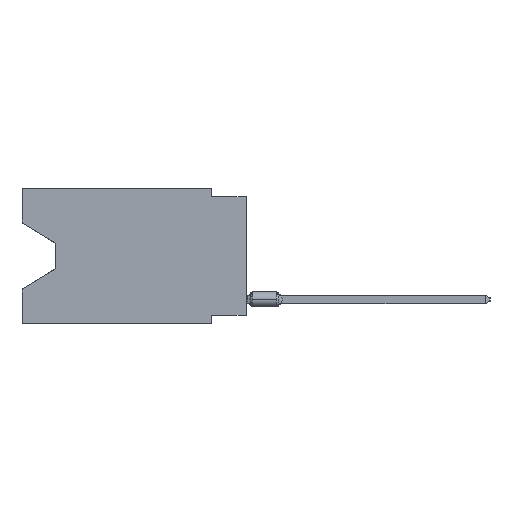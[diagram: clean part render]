
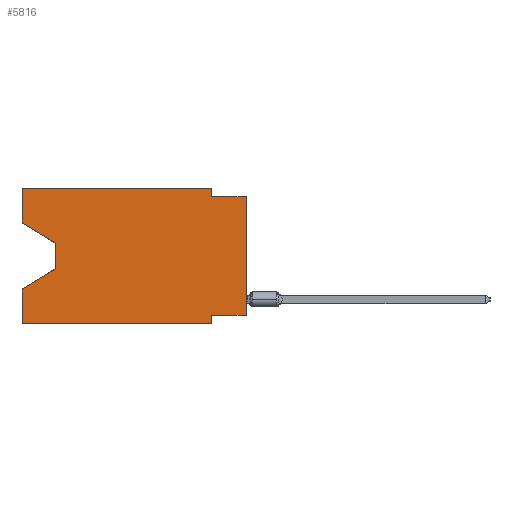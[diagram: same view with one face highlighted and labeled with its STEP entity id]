
A CAD part, left-side view. The second image highlights one B-rep face of the part: STEP entity #5816.
In plain terms, the highlighted planar face has unit normal (-1, 0, 0).
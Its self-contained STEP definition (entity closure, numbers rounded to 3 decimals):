
#464 = DIRECTION ( 'NONE',  ( 0., 1., 0. ) ) ;
#2467 = CARTESIAN_POINT ( 'NONE',  ( 0., 16.383, -9.906 ) ) ;
#3094 = VERTEX_POINT ( 'NONE', #14718 ) ;
#4189 = EDGE_CURVE ( 'NONE', #8635, #48757, #62027, .T. ) ;
#4239 = LINE ( 'NONE', #42988, #12880 ) ;
#5451 = VECTOR ( 'NONE', #45118, 1000. ) ;
#5816 = ADVANCED_FACE ( 'NONE', ( #43560 ), #16872, .F. ) ;
#7250 = DIRECTION ( 'NONE',  ( 0., 0., -1. ) ) ;
#7981 = CARTESIAN_POINT ( 'NONE',  ( 0., 16.383, 0. ) ) ;
#8635 = VERTEX_POINT ( 'NONE', #2467 ) ;
#9664 = EDGE_CURVE ( 'NONE', #64822, #18568, #26777, .T. ) ;
#10467 = EDGE_CURVE ( 'NONE', #55647, #65699, #4239, .T. ) ;
#11628 = ORIENTED_EDGE ( 'NONE', *, *, #9664, .F. ) ;
#11661 = CARTESIAN_POINT ( 'NONE',  ( 0., 0., -9.271 ) ) ;
#12830 = CARTESIAN_POINT ( 'NONE',  ( 0., 2.54, 0. ) ) ;
#12880 = VECTOR ( 'NONE', #19888, 1000. ) ;
#12943 = LINE ( 'NONE', #44962, #26916 ) ;
#13711 = EDGE_CURVE ( 'NONE', #25916, #25682, #12943, .T. ) ;
#13853 = VECTOR ( 'NONE', #7250, 1000. ) ;
#14541 = DIRECTION ( 'NONE',  ( 0., -1., 0. ) ) ;
#14718 = CARTESIAN_POINT ( 'NONE',  ( 0., 0., -0.635 ) ) ;
#16023 = ORIENTED_EDGE ( 'NONE', *, *, #34497, .F. ) ;
#16143 = VECTOR ( 'NONE', #464, 1000. ) ;
#16872 = PLANE ( 'NONE',  #20350 ) ;
#17101 = DIRECTION ( 'NONE',  ( 0., 0., 1. ) ) ;
#17209 = EDGE_CURVE ( 'NONE', #20683, #25916, #69921, .T. ) ;
#18568 = VERTEX_POINT ( 'NONE', #43500 ) ;
#19888 = DIRECTION ( 'NONE',  ( 0., -0.855, -0.519 ) ) ;
#20350 = AXIS2_PLACEMENT_3D ( 'NONE', #65239, #43205, #44271 ) ;
#20374 = VERTEX_POINT ( 'NONE', #68039 ) ;
#20683 = VERTEX_POINT ( 'NONE', #30255 ) ;
#22502 = DIRECTION ( 'NONE',  ( 0., 0.855, -0.519 ) ) ;
#23044 = CARTESIAN_POINT ( 'NONE',  ( 0., 16.383, 0. ) ) ;
#23615 = DIRECTION ( 'NONE',  ( 0., 0., 1. ) ) ;
#24322 = CARTESIAN_POINT ( 'NONE',  ( 0., 13.97, -5.893 ) ) ;
#24581 = EDGE_CURVE ( 'NONE', #64822, #3094, #64392, .T. ) ;
#25393 = VECTOR ( 'NONE', #14541, 1000. ) ;
#25682 = VERTEX_POINT ( 'NONE', #31022 ) ;
#25916 = VERTEX_POINT ( 'NONE', #12830 ) ;
#26777 = LINE ( 'NONE', #43155, #16143 ) ;
#26916 = VECTOR ( 'NONE', #60928, 1000. ) ;
#27500 = CARTESIAN_POINT ( 'NONE',  ( 0., 13.97, -5.893 ) ) ;
#27849 = LINE ( 'NONE', #27500, #65880 ) ;
#28495 = LINE ( 'NONE', #44164, #51606 ) ;
#30255 = CARTESIAN_POINT ( 'NONE',  ( 0., 16.383, 0. ) ) ;
#30617 = ORIENTED_EDGE ( 'NONE', *, *, #54413, .T. ) ;
#30844 = EDGE_CURVE ( 'NONE', #55647, #20683, #44427, .T. ) ;
#31022 = CARTESIAN_POINT ( 'NONE',  ( 0., 2.54, -0.635 ) ) ;
#33171 = ORIENTED_EDGE ( 'NONE', *, *, #60723, .T. ) ;
#33438 = CARTESIAN_POINT ( 'NONE',  ( 0., 13.97, -4.013 ) ) ;
#34497 = EDGE_CURVE ( 'NONE', #18568, #20374, #62003, .T. ) ;
#35001 = CARTESIAN_POINT ( 'NONE',  ( 0., 2.54, -9.906 ) ) ;
#35227 = VECTOR ( 'NONE', #42898, 1000. ) ;
#35434 = ORIENTED_EDGE ( 'NONE', *, *, #48854, .T. ) ;
#36892 = VECTOR ( 'NONE', #17101, 1000. ) ;
#37412 = LINE ( 'NONE', #38466, #69064 ) ;
#38466 = CARTESIAN_POINT ( 'NONE',  ( 0., 0., -0.635 ) ) ;
#41793 = VECTOR ( 'NONE', #23615, 1000. ) ;
#41878 = ORIENTED_EDGE ( 'NONE', *, *, #24581, .T. ) ;
#42898 = DIRECTION ( 'NONE',  ( 0., -1., 0. ) ) ;
#42988 = CARTESIAN_POINT ( 'NONE',  ( 0., 16.383, -2.546 ) ) ;
#43155 = CARTESIAN_POINT ( 'NONE',  ( 0., 0., -9.271 ) ) ;
#43205 = DIRECTION ( 'NONE',  ( 1., 0., 0. ) ) ;
#43500 = CARTESIAN_POINT ( 'NONE',  ( 0., 2.54, -9.271 ) ) ;
#43560 = FACE_OUTER_BOUND ( 'NONE', #46177, .T. ) ;
#44164 = CARTESIAN_POINT ( 'NONE',  ( 0., 13.97, -4.013 ) ) ;
#44271 = DIRECTION ( 'NONE',  ( 0., 0., -1. ) ) ;
#44427 = LINE ( 'NONE', #23044, #5451 ) ;
#44962 = CARTESIAN_POINT ( 'NONE',  ( 0., 2.54, 0. ) ) ;
#45118 = DIRECTION ( 'NONE',  ( 0., 0., 1. ) ) ;
#46177 = EDGE_LOOP ( 'NONE', ( #59662, #35434, #33171, #69735, #30617, #16023, #11628, #41878, #66070, #47464, #59280, #64768 ) ) ;
#46192 = VERTEX_POINT ( 'NONE', #24322 ) ;
#47464 = ORIENTED_EDGE ( 'NONE', *, *, #13711, .F. ) ;
#48757 = VERTEX_POINT ( 'NONE', #49845 ) ;
#48793 = DIRECTION ( 'NONE',  ( 0., -1., 0. ) ) ;
#48854 = EDGE_CURVE ( 'NONE', #65699, #46192, #28495, .T. ) ;
#49845 = CARTESIAN_POINT ( 'NONE',  ( 0., 16.383, -7.36 ) ) ;
#51606 = VECTOR ( 'NONE', #65846, 1000. ) ;
#52076 = EDGE_CURVE ( 'NONE', #25682, #3094, #37412, .T. ) ;
#53276 = LINE ( 'NONE', #53614, #25393 ) ;
#53614 = CARTESIAN_POINT ( 'NONE',  ( 0., 16.383, -9.906 ) ) ;
#54413 = EDGE_CURVE ( 'NONE', #8635, #20374, #53276, .T. ) ;
#54418 = CARTESIAN_POINT ( 'NONE',  ( 0., 0., 0. ) ) ;
#55647 = VERTEX_POINT ( 'NONE', #66467 ) ;
#58531 = CARTESIAN_POINT ( 'NONE',  ( 0., 16.383, 0. ) ) ;
#59280 = ORIENTED_EDGE ( 'NONE', *, *, #17209, .F. ) ;
#59662 = ORIENTED_EDGE ( 'NONE', *, *, #10467, .T. ) ;
#60723 = EDGE_CURVE ( 'NONE', #46192, #48757, #27849, .T. ) ;
#60928 = DIRECTION ( 'NONE',  ( 0., 0., -1. ) ) ;
#62003 = LINE ( 'NONE', #35001, #13853 ) ;
#62027 = LINE ( 'NONE', #7981, #41793 ) ;
#64392 = LINE ( 'NONE', #54418, #36892 ) ;
#64768 = ORIENTED_EDGE ( 'NONE', *, *, #30844, .F. ) ;
#64822 = VERTEX_POINT ( 'NONE', #11661 ) ;
#65239 = CARTESIAN_POINT ( 'NONE',  ( 0., 16.383, 0. ) ) ;
#65699 = VERTEX_POINT ( 'NONE', #33438 ) ;
#65846 = DIRECTION ( 'NONE',  ( 0., 0., -1. ) ) ;
#65880 = VECTOR ( 'NONE', #22502, 1000. ) ;
#66070 = ORIENTED_EDGE ( 'NONE', *, *, #52076, .F. ) ;
#66467 = CARTESIAN_POINT ( 'NONE',  ( 0., 16.383, -2.546 ) ) ;
#68039 = CARTESIAN_POINT ( 'NONE',  ( 0., 2.54, -9.906 ) ) ;
#69064 = VECTOR ( 'NONE', #48793, 1000. ) ;
#69735 = ORIENTED_EDGE ( 'NONE', *, *, #4189, .F. ) ;
#69921 = LINE ( 'NONE', #58531, #35227 ) ;
